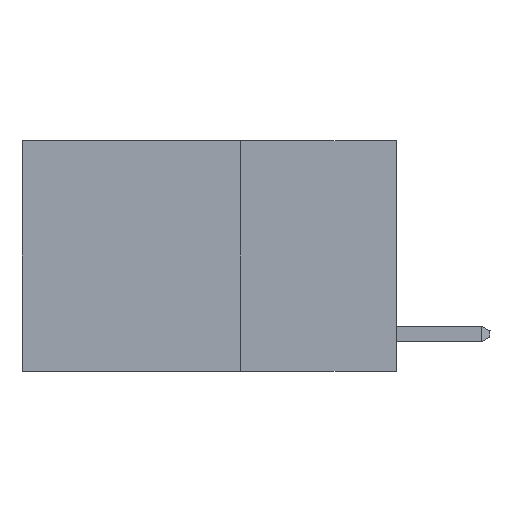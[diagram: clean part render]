
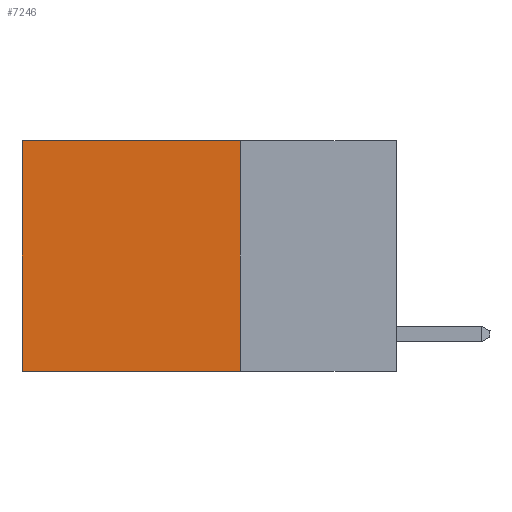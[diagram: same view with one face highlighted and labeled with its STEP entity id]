
A CAD part, left-side view. The second image highlights one B-rep face of the part: STEP entity #7246.
In plain terms, the highlighted planar face has unit normal (-1, 0, 0).
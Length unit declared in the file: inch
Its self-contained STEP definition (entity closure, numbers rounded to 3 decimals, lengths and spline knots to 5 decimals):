
#207 = CARTESIAN_POINT ( 'NONE',  ( 0.2625, 0.25, 0. ) ) ;
#297 = CARTESIAN_POINT ( 'NONE',  ( 0.2625, 0.6, -0.37 ) ) ;
#315 = VERTEX_POINT ( 'NONE', #2446 ) ;
#572 = DIRECTION ( 'NONE',  ( 1., 0., 0. ) ) ;
#789 = ORIENTED_EDGE ( 'NONE', *, *, #8254, .F. ) ;
#882 = ORIENTED_EDGE ( 'NONE', *, *, #7381, .T. ) ;
#1249 = AXIS2_PLACEMENT_3D ( 'NONE', #9419, #572, #7850 ) ;
#1587 = LINE ( 'NONE', #7527, #1701 ) ;
#1701 = VECTOR ( 'NONE', #5465, 39.37008 ) ;
#2220 = LINE ( 'NONE', #207, #7638 ) ;
#2327 = VERTEX_POINT ( 'NONE', #8995 ) ;
#2409 = CARTESIAN_POINT ( 'NONE',  ( 0.2625, 0.25, 0. ) ) ;
#2446 = CARTESIAN_POINT ( 'NONE',  ( 0.2625, 0.25, -0.37 ) ) ;
#2506 = EDGE_LOOP ( 'NONE', ( #882, #3545, #789, #2664 ) ) ;
#2635 = VERTEX_POINT ( 'NONE', #2409 ) ;
#2663 = VECTOR ( 'NONE', #6634, 39.37008 ) ;
#2664 = ORIENTED_EDGE ( 'NONE', *, *, #3415, .T. ) ;
#3137 = VERTEX_POINT ( 'NONE', #297 ) ;
#3148 = VECTOR ( 'NONE', #7403, 39.37008 ) ;
#3415 = EDGE_CURVE ( 'NONE', #2635, #2327, #2220, .T. ) ;
#3545 = ORIENTED_EDGE ( 'NONE', *, *, #8037, .F. ) ;
#5330 = DIRECTION ( 'NONE',  ( 0., 1., 0. ) ) ;
#5465 = DIRECTION ( 'NONE',  ( 0., 0., -1. ) ) ;
#6151 = LINE ( 'NONE', #7371, #3148 ) ;
#6255 = FACE_OUTER_BOUND ( 'NONE', #2506, .T. ) ;
#6634 = DIRECTION ( 'NONE',  ( 0., 1., 0. ) ) ;
#7246 = ADVANCED_FACE ( 'NONE', ( #6255 ), #7271, .F. ) ;
#7271 = PLANE ( 'NONE',  #1249 ) ;
#7367 = LINE ( 'NONE', #7422, #2663 ) ;
#7371 = CARTESIAN_POINT ( 'NONE',  ( 0.2625, 0.6, 0. ) ) ;
#7381 = EDGE_CURVE ( 'NONE', #2327, #3137, #6151, .T. ) ;
#7403 = DIRECTION ( 'NONE',  ( 0., 0., -1. ) ) ;
#7422 = CARTESIAN_POINT ( 'NONE',  ( 0.2625, 0.25, -0.37 ) ) ;
#7527 = CARTESIAN_POINT ( 'NONE',  ( 0.2625, 0.25, 0. ) ) ;
#7638 = VECTOR ( 'NONE', #5330, 39.37008 ) ;
#7850 = DIRECTION ( 'NONE',  ( 0., 0., -1. ) ) ;
#8037 = EDGE_CURVE ( 'NONE', #315, #3137, #7367, .T. ) ;
#8254 = EDGE_CURVE ( 'NONE', #2635, #315, #1587, .T. ) ;
#8995 = CARTESIAN_POINT ( 'NONE',  ( 0.2625, 0.6, 0. ) ) ;
#9419 = CARTESIAN_POINT ( 'NONE',  ( 0.2625, 0.25, 0. ) ) ;
